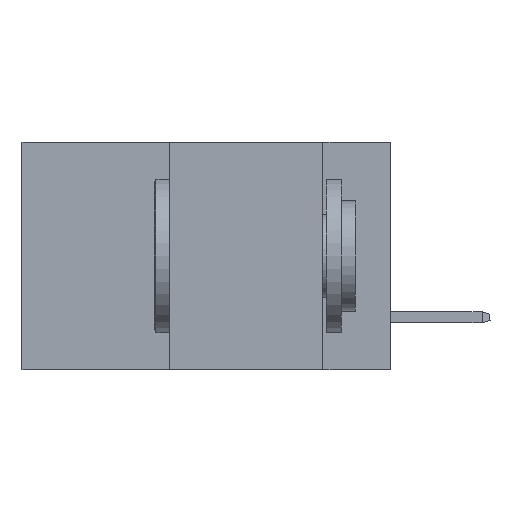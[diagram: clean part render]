
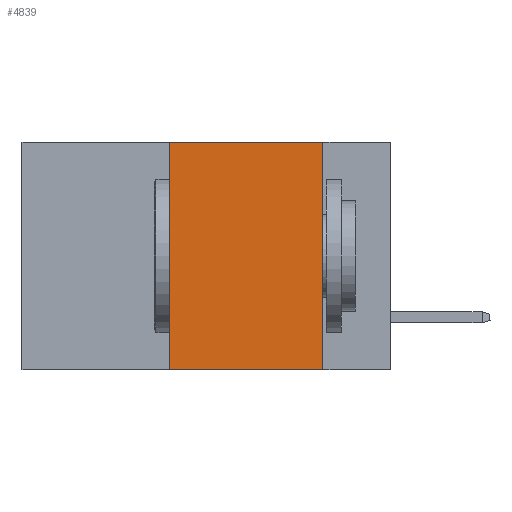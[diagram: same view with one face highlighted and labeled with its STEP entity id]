
A CAD part, left-side view. The second image highlights one B-rep face of the part: STEP entity #4839.
In plain terms, the highlighted planar face has unit normal (-1, 0, 0).
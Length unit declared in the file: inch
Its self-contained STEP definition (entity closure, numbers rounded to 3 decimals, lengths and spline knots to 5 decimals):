
#49 = CARTESIAN_POINT ( 'NONE',  ( 0., 0.36, 0. ) ) ;
#229 = EDGE_CURVE ( 'NONE', #9034, #7806, #933, .T. ) ;
#889 = EDGE_CURVE ( 'NONE', #11688, #8026, #6259, .T. ) ;
#933 = LINE ( 'NONE', #49, #12687 ) ;
#1039 = EDGE_CURVE ( 'NONE', #9034, #8026, #10151, .T. ) ;
#1405 = VECTOR ( 'NONE', #9141, 39.37008 ) ;
#1587 = DIRECTION ( 'NONE',  ( 1., 0., 0. ) ) ;
#1824 = CARTESIAN_POINT ( 'NONE',  ( 0., 0.6, -0.37 ) ) ;
#1835 = ORIENTED_EDGE ( 'NONE', *, *, #7482, .F. ) ;
#2750 = LINE ( 'NONE', #4906, #1405 ) ;
#2881 = ORIENTED_EDGE ( 'NONE', *, *, #889, .F. ) ;
#4839 = ADVANCED_FACE ( 'NONE', ( #13035 ), #5921, .F. ) ;
#4906 = CARTESIAN_POINT ( 'NONE',  ( 0., 0.6, 0. ) ) ;
#5921 = PLANE ( 'NONE',  #8265 ) ;
#6259 = LINE ( 'NONE', #6662, #12498 ) ;
#6396 = ORIENTED_EDGE ( 'NONE', *, *, #1039, .T. ) ;
#6662 = CARTESIAN_POINT ( 'NONE',  ( 0., 0.11, 0. ) ) ;
#7197 = EDGE_LOOP ( 'NONE', ( #2881, #1835, #11999, #6396 ) ) ;
#7277 = VECTOR ( 'NONE', #12566, 39.37008 ) ;
#7445 = CARTESIAN_POINT ( 'NONE',  ( 0., 0.36, -0.37 ) ) ;
#7482 = EDGE_CURVE ( 'NONE', #7806, #11688, #2750, .T. ) ;
#7806 = VERTEX_POINT ( 'NONE', #7837 ) ;
#7837 = CARTESIAN_POINT ( 'NONE',  ( 0., 0.36, 0. ) ) ;
#8026 = VERTEX_POINT ( 'NONE', #9696 ) ;
#8265 = AXIS2_PLACEMENT_3D ( 'NONE', #13534, #1587, #9097 ) ;
#8572 = DIRECTION ( 'NONE',  ( 0., 0., 1. ) ) ;
#9034 = VERTEX_POINT ( 'NONE', #7445 ) ;
#9097 = DIRECTION ( 'NONE',  ( 0., 0., -1. ) ) ;
#9141 = DIRECTION ( 'NONE',  ( 0., -1., 0. ) ) ;
#9696 = CARTESIAN_POINT ( 'NONE',  ( 0., 0.11, -0.37 ) ) ;
#10151 = LINE ( 'NONE', #1824, #7277 ) ;
#11183 = CARTESIAN_POINT ( 'NONE',  ( 0., 0.11, 0. ) ) ;
#11688 = VERTEX_POINT ( 'NONE', #11183 ) ;
#11999 = ORIENTED_EDGE ( 'NONE', *, *, #229, .F. ) ;
#12498 = VECTOR ( 'NONE', #13415, 39.37008 ) ;
#12566 = DIRECTION ( 'NONE',  ( 0., -1., 0. ) ) ;
#12687 = VECTOR ( 'NONE', #8572, 39.37008 ) ;
#13035 = FACE_OUTER_BOUND ( 'NONE', #7197, .T. ) ;
#13415 = DIRECTION ( 'NONE',  ( 0., 0., -1. ) ) ;
#13534 = CARTESIAN_POINT ( 'NONE',  ( 0., 0.6, 0. ) ) ;
